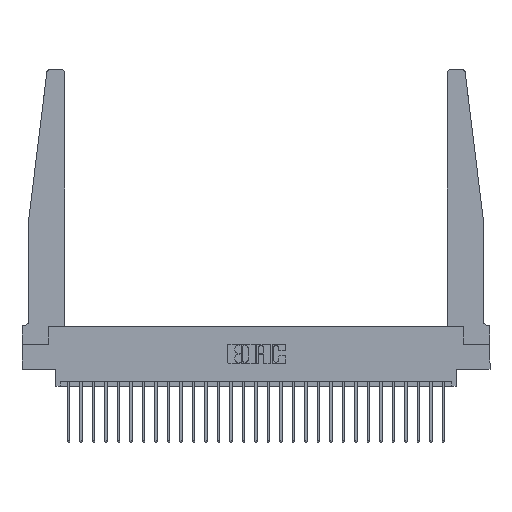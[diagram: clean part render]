
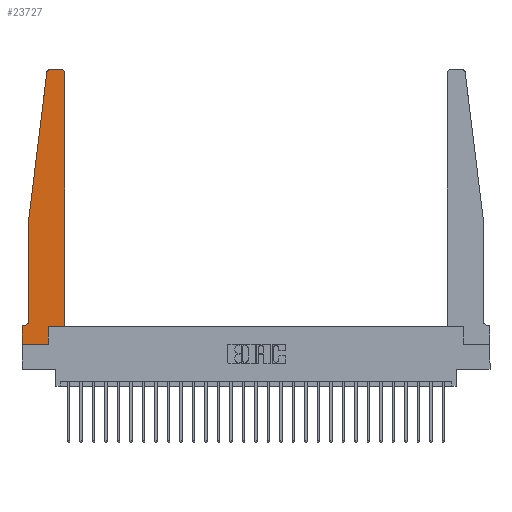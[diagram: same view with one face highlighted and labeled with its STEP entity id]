
A CAD part, top view. The second image highlights one B-rep face of the part: STEP entity #23727.
In plain terms, the highlighted planar face has unit normal (0, 0, 1).
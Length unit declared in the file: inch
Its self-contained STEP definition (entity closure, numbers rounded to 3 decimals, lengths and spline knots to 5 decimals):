
#48 = DIRECTION ( 'NONE',  ( 1., 0., 0. ) ) ;
#255 = AXIS2_PLACEMENT_3D ( 'NONE', #7962, #22407, #10029 ) ;
#543 = ORIENTED_EDGE ( 'NONE', *, *, #12842, .T. ) ;
#1204 = VECTOR ( 'NONE', #11337, 39.37008 ) ;
#1387 = EDGE_CURVE ( 'NONE', #8872, #3126, #7033, .T. ) ;
#1538 = EDGE_CURVE ( 'NONE', #20738, #25244, #25137, .T. ) ;
#1595 = ORIENTED_EDGE ( 'NONE', *, *, #9595, .T. ) ;
#1732 = CARTESIAN_POINT ( 'NONE',  ( 0.25, 2.75, 0.37 ) ) ;
#2344 = CIRCLE ( 'NONE', #13931, 0.03 ) ;
#2403 = CARTESIAN_POINT ( 'NONE',  ( 0.425, 0.18, 0.37 ) ) ;
#2955 = LINE ( 'NONE', #21971, #24226 ) ;
#3126 = VERTEX_POINT ( 'NONE', #17717 ) ;
#3279 = LINE ( 'NONE', #17101, #14845 ) ;
#3501 = ORIENTED_EDGE ( 'NONE', *, *, #24846, .T. ) ;
#4272 = CARTESIAN_POINT ( 'NONE',  ( 0.015, 0.2375, 0.37 ) ) ;
#4546 = DIRECTION ( 'NONE',  ( -1., 0., 0. ) ) ;
#4763 = DIRECTION ( 'NONE',  ( 0., -1., 0. ) ) ;
#4765 = ORIENTED_EDGE ( 'NONE', *, *, #18059, .T. ) ;
#4818 = ORIENTED_EDGE ( 'NONE', *, *, #9400, .T. ) ;
#5101 = EDGE_CURVE ( 'NONE', #20343, #6250, #16858, .T. ) ;
#5197 = CARTESIAN_POINT ( 'NONE',  ( 0.24675, 2.72367, 0.37 ) ) ;
#6217 = VECTOR ( 'NONE', #16736, 39.37008 ) ;
#6250 = VERTEX_POINT ( 'NONE', #25902 ) ;
#6319 = DIRECTION ( 'NONE',  ( -1., 0., 0. ) ) ;
#6322 = CARTESIAN_POINT ( 'NONE',  ( 0.395, 2.75, 0.37 ) ) ;
#6350 = CARTESIAN_POINT ( 'NONE',  ( 0.065, 1.25, 0.37 ) ) ;
#6473 = DIRECTION ( 'NONE',  ( 0., 0., 1. ) ) ;
#6714 = CARTESIAN_POINT ( 'NONE',  ( 0.065, 0.2375, 0.37 ) ) ;
#7033 = LINE ( 'NONE', #1732, #22861 ) ;
#7962 = CARTESIAN_POINT ( 'NONE',  ( 0., 0.1875, 0.37 ) ) ;
#7988 = CIRCLE ( 'NONE', #13655, 0.05 ) ;
#8298 = ORIENTED_EDGE ( 'NONE', *, *, #1538, .T. ) ;
#8872 = VERTEX_POINT ( 'NONE', #6322 ) ;
#8929 = VERTEX_POINT ( 'NONE', #2403 ) ;
#9400 = EDGE_CURVE ( 'NONE', #12479, #8872, #2344, .T. ) ;
#9589 = ORIENTED_EDGE ( 'NONE', *, *, #5101, .T. ) ;
#9595 = EDGE_CURVE ( 'NONE', #25336, #13824, #3279, .T. ) ;
#9887 = CARTESIAN_POINT ( 'NONE',  ( 0.2605, 0.18, 0.37 ) ) ;
#10029 = DIRECTION ( 'NONE',  ( 1., 0., 0. ) ) ;
#10587 = CARTESIAN_POINT ( 'NONE',  ( 0.425, 0.18, 0.37 ) ) ;
#11121 = DIRECTION ( 'NONE',  ( 1., 0., 0. ) ) ;
#11337 = DIRECTION ( 'NONE',  ( -0.122, -0.992, 0. ) ) ;
#11934 = DIRECTION ( 'NONE',  ( 0., 1., 0. ) ) ;
#12308 = DIRECTION ( 'NONE',  ( 0., 0., 1. ) ) ;
#12479 = VERTEX_POINT ( 'NONE', #19296 ) ;
#12697 = CARTESIAN_POINT ( 'NONE',  ( 0.065, 0.1875, 0.37 ) ) ;
#12842 = EDGE_CURVE ( 'NONE', #21410, #25336, #16933, .T. ) ;
#13455 = VECTOR ( 'NONE', #4546, 39.37008 ) ;
#13655 = AXIS2_PLACEMENT_3D ( 'NONE', #4272, #18694, #6319 ) ;
#13703 = DIRECTION ( 'NONE',  ( 1., 0., 0. ) ) ;
#13824 = VERTEX_POINT ( 'NONE', #6714 ) ;
#13931 = AXIS2_PLACEMENT_3D ( 'NONE', #24725, #12308, #48 ) ;
#14270 = LINE ( 'NONE', #26165, #21202 ) ;
#14762 = EDGE_CURVE ( 'NONE', #25244, #21638, #14270, .T. ) ;
#14845 = VECTOR ( 'NONE', #4763, 39.37008 ) ;
#16059 = CIRCLE ( 'NONE', #19908, 0.03 ) ;
#16070 = DIRECTION ( 'NONE',  ( -1., 0., 0. ) ) ;
#16115 = FACE_OUTER_BOUND ( 'NONE', #22064, .T. ) ;
#16274 = ORIENTED_EDGE ( 'NONE', *, *, #24652, .T. ) ;
#16736 = DIRECTION ( 'NONE',  ( 0., 1., 0. ) ) ;
#16858 = LINE ( 'NONE', #9887, #21072 ) ;
#16933 = LINE ( 'NONE', #25808, #1204 ) ;
#17101 = CARTESIAN_POINT ( 'NONE',  ( 0.065, 1.25, 0.37 ) ) ;
#17717 = CARTESIAN_POINT ( 'NONE',  ( 0.27653, 2.75, 0.37 ) ) ;
#18059 = EDGE_CURVE ( 'NONE', #8929, #12479, #22688, .T. ) ;
#18157 = PLANE ( 'NONE',  #255 ) ;
#18694 = DIRECTION ( 'NONE',  ( 0., 0., -1. ) ) ;
#18715 = VECTOR ( 'NONE', #11121, 39.37008 ) ;
#18854 = CARTESIAN_POINT ( 'NONE',  ( 0.27653, 2.72, 0.37 ) ) ;
#19282 = ORIENTED_EDGE ( 'NONE', *, *, #14762, .T. ) ;
#19296 = CARTESIAN_POINT ( 'NONE',  ( 0.425, 2.72, 0.37 ) ) ;
#19300 = CARTESIAN_POINT ( 'NONE',  ( 0.015, 0.1875, 0.37 ) ) ;
#19908 = AXIS2_PLACEMENT_3D ( 'NONE', #18854, #6473, #20924 ) ;
#20042 = DIRECTION ( 'NONE',  ( 0., -1., 0. ) ) ;
#20343 = VERTEX_POINT ( 'NONE', #26176 ) ;
#20536 = CARTESIAN_POINT ( 'NONE',  ( 0., 0.1875, 0.37 ) ) ;
#20592 = ORIENTED_EDGE ( 'NONE', *, *, #23610, .T. ) ;
#20738 = VERTEX_POINT ( 'NONE', #19300 ) ;
#20924 = DIRECTION ( 'NONE',  ( 1., 0., 0. ) ) ;
#21072 = VECTOR ( 'NONE', #11934, 39.37008 ) ;
#21138 = ORIENTED_EDGE ( 'NONE', *, *, #1387, .T. ) ;
#21202 = VECTOR ( 'NONE', #20042, 39.37008 ) ;
#21410 = VERTEX_POINT ( 'NONE', #5197 ) ;
#21638 = VERTEX_POINT ( 'NONE', #22428 ) ;
#21971 = CARTESIAN_POINT ( 'NONE',  ( 0.425, 0.18, 0.37 ) ) ;
#22064 = EDGE_LOOP ( 'NONE', ( #21138, #16274, #543, #1595, #23483, #8298, #19282, #3501, #9589, #20592, #4765, #4818 ) ) ;
#22407 = DIRECTION ( 'NONE',  ( 0., 0., 1. ) ) ;
#22428 = CARTESIAN_POINT ( 'NONE',  ( 0., 0., 0.37 ) ) ;
#22688 = LINE ( 'NONE', #10587, #6217 ) ;
#22861 = VECTOR ( 'NONE', #16070, 39.37008 ) ;
#23483 = ORIENTED_EDGE ( 'NONE', *, *, #26012, .T. ) ;
#23610 = EDGE_CURVE ( 'NONE', #6250, #8929, #2955, .T. ) ;
#23727 = ADVANCED_FACE ( 'NONE', ( #16115 ), #18157, .T. ) ;
#24210 = LINE ( 'NONE', #25606, #18715 ) ;
#24226 = VECTOR ( 'NONE', #13703, 39.37008 ) ;
#24652 = EDGE_CURVE ( 'NONE', #3126, #21410, #16059, .T. ) ;
#24725 = CARTESIAN_POINT ( 'NONE',  ( 0.395, 2.72, 0.37 ) ) ;
#24846 = EDGE_CURVE ( 'NONE', #21638, #20343, #24210, .T. ) ;
#25137 = LINE ( 'NONE', #12697, #13455 ) ;
#25244 = VERTEX_POINT ( 'NONE', #20536 ) ;
#25336 = VERTEX_POINT ( 'NONE', #6350 ) ;
#25606 = CARTESIAN_POINT ( 'NONE',  ( 0., 0., 0.37 ) ) ;
#25808 = CARTESIAN_POINT ( 'NONE',  ( 0.065, 1.25, 0.37 ) ) ;
#25902 = CARTESIAN_POINT ( 'NONE',  ( 0.2605, 0.18, 0.37 ) ) ;
#26012 = EDGE_CURVE ( 'NONE', #13824, #20738, #7988, .T. ) ;
#26165 = CARTESIAN_POINT ( 'NONE',  ( 0., 0., 0.37 ) ) ;
#26176 = CARTESIAN_POINT ( 'NONE',  ( 0.2605, 0., 0.37 ) ) ;
